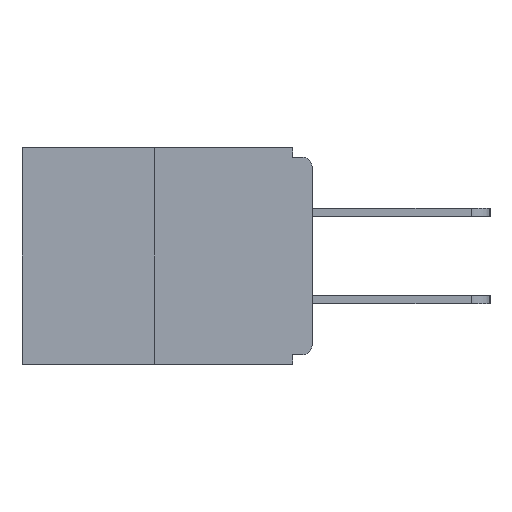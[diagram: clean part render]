
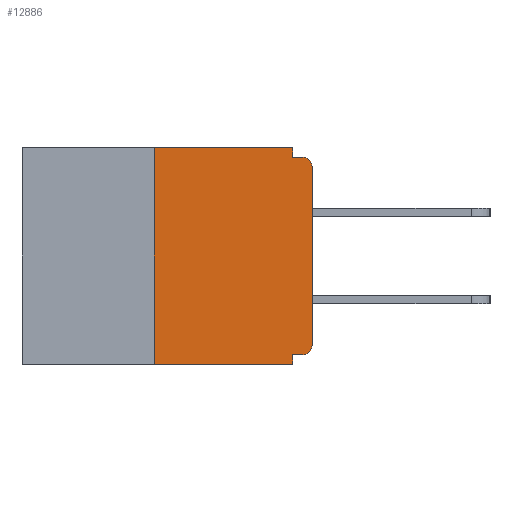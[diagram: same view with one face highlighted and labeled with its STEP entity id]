
A CAD part, left-side view. The second image highlights one B-rep face of the part: STEP entity #12886.
In plain terms, the highlighted planar face has unit normal (-1, 0, 0).
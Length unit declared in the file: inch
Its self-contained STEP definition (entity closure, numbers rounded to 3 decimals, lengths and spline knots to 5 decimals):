
#357 = EDGE_CURVE ( 'NONE', #18007, #8397, #13102, .T. ) ;
#363 = EDGE_LOOP ( 'NONE', ( #10686, #367, #5723, #6291, #13214, #17468, #14905, #5746, #19683, #11300 ) ) ;
#367 = ORIENTED_EDGE ( 'NONE', *, *, #17616, .F. ) ;
#463 = AXIS2_PLACEMENT_3D ( 'NONE', #17509, #19384, #9047 ) ;
#1103 = DIRECTION ( 'NONE',  ( -1., 0., 0. ) ) ;
#1467 = LINE ( 'NONE', #13128, #20838 ) ;
#1780 = VECTOR ( 'NONE', #7455, 39.37008 ) ;
#2003 = CARTESIAN_POINT ( 'NONE',  ( 0., 0.46, 0. ) ) ;
#2465 = AXIS2_PLACEMENT_3D ( 'NONE', #19861, #1103, #12992 ) ;
#2708 = LINE ( 'NONE', #21347, #1780 ) ;
#3010 = DIRECTION ( 'NONE',  ( 0., 0., -1. ) ) ;
#4140 = LINE ( 'NONE', #12935, #10406 ) ;
#4481 = LINE ( 'NONE', #17630, #8977 ) ;
#4957 = VERTEX_POINT ( 'NONE', #11133 ) ;
#5237 = DIRECTION ( 'NONE',  ( 0., 0., 1. ) ) ;
#5718 = EDGE_CURVE ( 'NONE', #20905, #10678, #4140, .T. ) ;
#5723 = ORIENTED_EDGE ( 'NONE', *, *, #17299, .T. ) ;
#5746 = ORIENTED_EDGE ( 'NONE', *, *, #16181, .T. ) ;
#6066 = CARTESIAN_POINT ( 'NONE',  ( 0., 0., 0. ) ) ;
#6097 = CIRCLE ( 'NONE', #463, 0.015 ) ;
#6227 = EDGE_CURVE ( 'NONE', #14890, #18258, #1467, .T. ) ;
#6291 = ORIENTED_EDGE ( 'NONE', *, *, #14419, .F. ) ;
#6877 = VERTEX_POINT ( 'NONE', #8812 ) ;
#7455 = DIRECTION ( 'NONE',  ( 0., -1., 0. ) ) ;
#7931 = CARTESIAN_POINT ( 'NONE',  ( 0., 0.031, 0. ) ) ;
#8323 = EDGE_CURVE ( 'NONE', #6877, #14890, #21191, .T. ) ;
#8397 = VERTEX_POINT ( 'NONE', #15422 ) ;
#8812 = CARTESIAN_POINT ( 'NONE',  ( 0., 0.25, 0. ) ) ;
#8977 = VECTOR ( 'NONE', #18067, 39.37008 ) ;
#9047 = DIRECTION ( 'NONE',  ( 0., 0., -1. ) ) ;
#9880 = CARTESIAN_POINT ( 'NONE',  ( 0., 0.031, -0.343 ) ) ;
#10023 = CARTESIAN_POINT ( 'NONE',  ( 0., 0.031, -0.328 ) ) ;
#10406 = VECTOR ( 'NONE', #21145, 39.37008 ) ;
#10485 = VECTOR ( 'NONE', #21413, 39.37008 ) ;
#10632 = CARTESIAN_POINT ( 'NONE',  ( 0., 0.031, -0.343 ) ) ;
#10678 = VERTEX_POINT ( 'NONE', #10023 ) ;
#10686 = ORIENTED_EDGE ( 'NONE', *, *, #8323, .F. ) ;
#11083 = DIRECTION ( 'NONE',  ( 0., 0., 1. ) ) ;
#11133 = CARTESIAN_POINT ( 'NONE',  ( 0., 0.015, -0.015 ) ) ;
#11300 = ORIENTED_EDGE ( 'NONE', *, *, #6227, .F. ) ;
#11307 = CARTESIAN_POINT ( 'NONE',  ( 0., 0.015, -0.328 ) ) ;
#11945 = VERTEX_POINT ( 'NONE', #13997 ) ;
#12744 = CARTESIAN_POINT ( 'NONE',  ( 0., 0.46, 0. ) ) ;
#12808 = VECTOR ( 'NONE', #19431, 39.37008 ) ;
#12886 = ADVANCED_FACE ( 'NONE', ( #17000 ), #20433, .F. ) ;
#12935 = CARTESIAN_POINT ( 'NONE',  ( 0., 0., -0.328 ) ) ;
#12992 = DIRECTION ( 'NONE',  ( 0., 0., -1. ) ) ;
#13102 = LINE ( 'NONE', #6066, #16533 ) ;
#13128 = CARTESIAN_POINT ( 'NONE',  ( 0., 0.031, 0. ) ) ;
#13214 = ORIENTED_EDGE ( 'NONE', *, *, #5718, .F. ) ;
#13281 = EDGE_CURVE ( 'NONE', #20905, #18007, #13487, .T. ) ;
#13487 = CIRCLE ( 'NONE', #2465, 0.015 ) ;
#13997 = CARTESIAN_POINT ( 'NONE',  ( 0., 0.25, -0.343 ) ) ;
#14042 = CARTESIAN_POINT ( 'NONE',  ( 0., 0.25, 0. ) ) ;
#14419 = EDGE_CURVE ( 'NONE', #10678, #18450, #19099, .T. ) ;
#14890 = VERTEX_POINT ( 'NONE', #7931 ) ;
#14905 = ORIENTED_EDGE ( 'NONE', *, *, #357, .T. ) ;
#15422 = CARTESIAN_POINT ( 'NONE',  ( 0., 0., -0.03 ) ) ;
#16181 = EDGE_CURVE ( 'NONE', #8397, #4957, #6097, .T. ) ;
#16359 = CARTESIAN_POINT ( 'NONE',  ( 0., 0., -0.313 ) ) ;
#16533 = VECTOR ( 'NONE', #11083, 39.37008 ) ;
#17000 = FACE_OUTER_BOUND ( 'NONE', #363, .T. ) ;
#17299 = EDGE_CURVE ( 'NONE', #11945, #18450, #4481, .T. ) ;
#17468 = ORIENTED_EDGE ( 'NONE', *, *, #13281, .T. ) ;
#17509 = CARTESIAN_POINT ( 'NONE',  ( 0., 0.015, -0.03 ) ) ;
#17616 = EDGE_CURVE ( 'NONE', #11945, #6877, #20477, .T. ) ;
#17630 = CARTESIAN_POINT ( 'NONE',  ( 0., 0.46, -0.343 ) ) ;
#17797 = EDGE_CURVE ( 'NONE', #18258, #4957, #2708, .T. ) ;
#18007 = VERTEX_POINT ( 'NONE', #16359 ) ;
#18067 = DIRECTION ( 'NONE',  ( 0., -1., 0. ) ) ;
#18258 = VERTEX_POINT ( 'NONE', #20782 ) ;
#18450 = VERTEX_POINT ( 'NONE', #9880 ) ;
#18656 = DIRECTION ( 'NONE',  ( 1., 0., 0. ) ) ;
#19099 = LINE ( 'NONE', #10632, #12808 ) ;
#19297 = VECTOR ( 'NONE', #5237, 39.37008 ) ;
#19384 = DIRECTION ( 'NONE',  ( -1., 0., 0. ) ) ;
#19431 = DIRECTION ( 'NONE',  ( 0., 0., -1. ) ) ;
#19683 = ORIENTED_EDGE ( 'NONE', *, *, #17797, .F. ) ;
#19861 = CARTESIAN_POINT ( 'NONE',  ( 0., 0.015, -0.313 ) ) ;
#20433 = PLANE ( 'NONE',  #21612 ) ;
#20477 = LINE ( 'NONE', #14042, #19297 ) ;
#20534 = DIRECTION ( 'NONE',  ( 0., 0., -1. ) ) ;
#20782 = CARTESIAN_POINT ( 'NONE',  ( 0., 0.031, -0.015 ) ) ;
#20838 = VECTOR ( 'NONE', #3010, 39.37008 ) ;
#20905 = VERTEX_POINT ( 'NONE', #11307 ) ;
#21145 = DIRECTION ( 'NONE',  ( 0., 1., 0. ) ) ;
#21191 = LINE ( 'NONE', #12744, #10485 ) ;
#21347 = CARTESIAN_POINT ( 'NONE',  ( 0., 0., -0.015 ) ) ;
#21413 = DIRECTION ( 'NONE',  ( 0., -1., 0. ) ) ;
#21612 = AXIS2_PLACEMENT_3D ( 'NONE', #2003, #18656, #20534 ) ;
